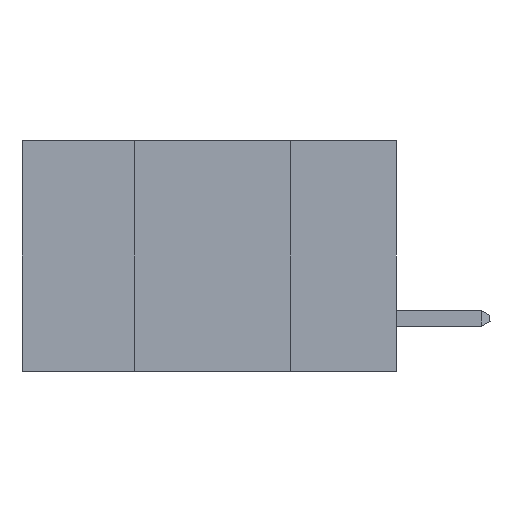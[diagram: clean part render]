
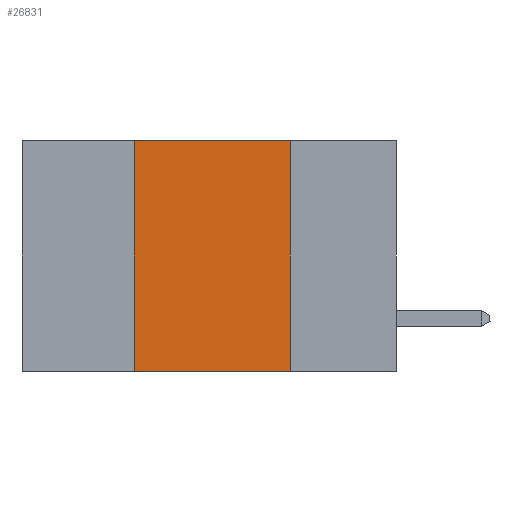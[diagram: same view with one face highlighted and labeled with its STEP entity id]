
A CAD part, left-side view. The second image highlights one B-rep face of the part: STEP entity #26831.
In plain terms, the highlighted planar face has unit normal (-1, 0, 0).
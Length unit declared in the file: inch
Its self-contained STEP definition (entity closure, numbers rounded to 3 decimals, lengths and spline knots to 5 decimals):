
#2581 = VERTEX_POINT ( 'NONE', #7279 ) ;
#4815 = ORIENTED_EDGE ( 'NONE', *, *, #30281, .F. ) ;
#6469 = PLANE ( 'NONE',  #22674 ) ;
#7279 = CARTESIAN_POINT ( 'NONE',  ( 0., 0.17, 0. ) ) ;
#7330 = LINE ( 'NONE', #24609, #13253 ) ;
#7839 = VERTEX_POINT ( 'NONE', #21507 ) ;
#9603 = ORIENTED_EDGE ( 'NONE', *, *, #12896, .F. ) ;
#11349 = VECTOR ( 'NONE', #19021, 39.37008 ) ;
#11368 = EDGE_LOOP ( 'NONE', ( #4815, #14764, #9603, #26416 ) ) ;
#11566 = DIRECTION ( 'NONE',  ( 1., 0., 0. ) ) ;
#11973 = EDGE_CURVE ( 'NONE', #7839, #2581, #7330, .T. ) ;
#12761 = VERTEX_POINT ( 'NONE', #27704 ) ;
#12896 = EDGE_CURVE ( 'NONE', #12761, #7839, #18394, .T. ) ;
#13253 = VECTOR ( 'NONE', #27202, 39.37008 ) ;
#14764 = ORIENTED_EDGE ( 'NONE', *, *, #11973, .F. ) ;
#16459 = CARTESIAN_POINT ( 'NONE',  ( 0., 0.6, -0.37 ) ) ;
#16964 = LINE ( 'NONE', #26061, #23775 ) ;
#18394 = LINE ( 'NONE', #31182, #24405 ) ;
#18404 = DIRECTION ( 'NONE',  ( 0., 0., 1. ) ) ;
#19021 = DIRECTION ( 'NONE',  ( 0., -1., 0. ) ) ;
#20908 = DIRECTION ( 'NONE',  ( 0., 0., -1. ) ) ;
#21507 = CARTESIAN_POINT ( 'NONE',  ( 0., 0.42, 0. ) ) ;
#22674 = AXIS2_PLACEMENT_3D ( 'NONE', #26893, #11566, #29465 ) ;
#23775 = VECTOR ( 'NONE', #20908, 39.37008 ) ;
#24405 = VECTOR ( 'NONE', #18404, 39.37008 ) ;
#24609 = CARTESIAN_POINT ( 'NONE',  ( 0., 0.6, 0. ) ) ;
#24948 = LINE ( 'NONE', #16459, #11349 ) ;
#26061 = CARTESIAN_POINT ( 'NONE',  ( 0., 0.17, 0. ) ) ;
#26416 = ORIENTED_EDGE ( 'NONE', *, *, #31803, .T. ) ;
#26679 = CARTESIAN_POINT ( 'NONE',  ( 0., 0.17, -0.37 ) ) ;
#26831 = ADVANCED_FACE ( 'NONE', ( #32444 ), #6469, .F. ) ;
#26893 = CARTESIAN_POINT ( 'NONE',  ( 0., 0.6, 0. ) ) ;
#27202 = DIRECTION ( 'NONE',  ( 0., -1., 0. ) ) ;
#27704 = CARTESIAN_POINT ( 'NONE',  ( 0., 0.42, -0.37 ) ) ;
#29465 = DIRECTION ( 'NONE',  ( 0., 0., -1. ) ) ;
#30281 = EDGE_CURVE ( 'NONE', #2581, #31122, #16964, .T. ) ;
#31122 = VERTEX_POINT ( 'NONE', #26679 ) ;
#31182 = CARTESIAN_POINT ( 'NONE',  ( 0., 0.42, 0. ) ) ;
#31803 = EDGE_CURVE ( 'NONE', #12761, #31122, #24948, .T. ) ;
#32444 = FACE_OUTER_BOUND ( 'NONE', #11368, .T. ) ;
